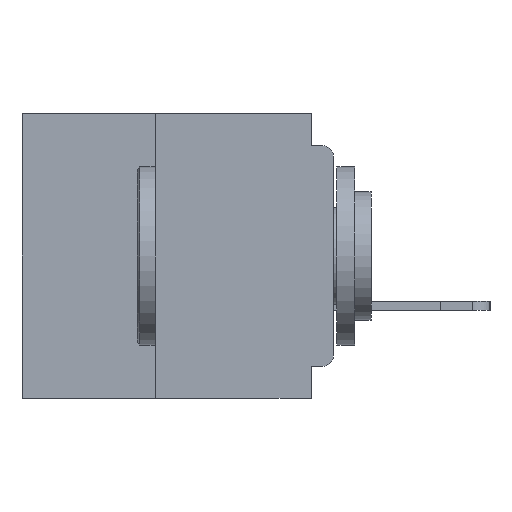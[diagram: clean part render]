
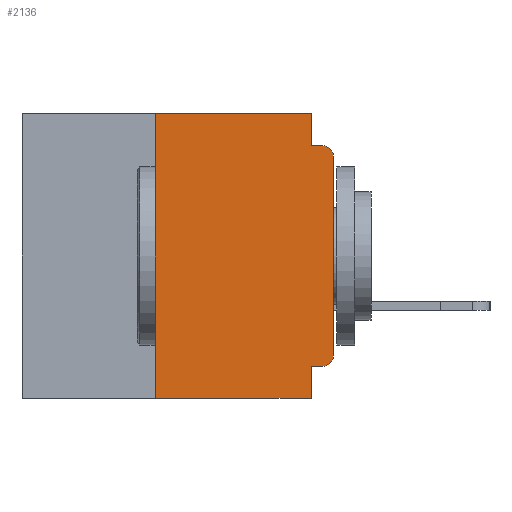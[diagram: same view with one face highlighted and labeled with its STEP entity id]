
A CAD part, left-side view. The second image highlights one B-rep face of the part: STEP entity #2136.
In plain terms, the highlighted planar face has unit normal (-1, 0, 0).
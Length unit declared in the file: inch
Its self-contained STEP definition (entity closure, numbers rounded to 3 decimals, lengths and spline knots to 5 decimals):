
#831 = LINE ( 'NONE', #15381, #50218 ) ;
#1664 = EDGE_CURVE ( 'NONE', #14596, #16155, #32058, .T. ) ;
#2136 = ADVANCED_FACE ( 'NONE', ( #37481 ), #32467, .F. ) ;
#2362 = VERTEX_POINT ( 'NONE', #25327 ) ;
#2366 = CARTESIAN_POINT ( 'NONE',  ( 0., 0.015, -0.355 ) ) ;
#2578 = EDGE_CURVE ( 'NONE', #16155, #28811, #19187, .T. ) ;
#3343 = AXIS2_PLACEMENT_3D ( 'NONE', #37265, #13981, #41214 ) ;
#3678 = ORIENTED_EDGE ( 'NONE', *, *, #29369, .F. ) ;
#4217 = VECTOR ( 'NONE', #15801, 39.37008 ) ;
#6455 = EDGE_CURVE ( 'NONE', #28859, #28811, #13585, .T. ) ;
#6988 = EDGE_CURVE ( 'NONE', #14596, #2362, #22668, .T. ) ;
#7192 = ORIENTED_EDGE ( 'NONE', *, *, #6988, .T. ) ;
#7932 = CARTESIAN_POINT ( 'NONE',  ( 0., 0., 0. ) ) ;
#10696 = CARTESIAN_POINT ( 'NONE',  ( 0., 0.25, 0. ) ) ;
#10801 = VERTEX_POINT ( 'NONE', #24145 ) ;
#12001 = CARTESIAN_POINT ( 'NONE',  ( 0., 0.031, -0.045 ) ) ;
#12273 = DIRECTION ( 'NONE',  ( 0., 0., 1. ) ) ;
#12374 = CARTESIAN_POINT ( 'NONE',  ( 0., 0.031, -0.355 ) ) ;
#12497 = VERTEX_POINT ( 'NONE', #31125 ) ;
#13357 = DIRECTION ( 'NONE',  ( 0., -1., 0. ) ) ;
#13410 = ORIENTED_EDGE ( 'NONE', *, *, #27637, .T. ) ;
#13585 = LINE ( 'NONE', #45611, #16021 ) ;
#13981 = DIRECTION ( 'NONE',  ( -1., 0., 0. ) ) ;
#13980 = VECTOR ( 'NONE', #22841, 39.37008 ) ;
#14596 = VERTEX_POINT ( 'NONE', #2366 ) ;
#14683 = LINE ( 'NONE', #7932, #4217 ) ;
#14730 = ORIENTED_EDGE ( 'NONE', *, *, #19282, .T. ) ;
#14836 = CARTESIAN_POINT ( 'NONE',  ( 0., 0.031, -0.4 ) ) ;
#15078 = ORIENTED_EDGE ( 'NONE', *, *, #1664, .F. ) ;
#15176 = CARTESIAN_POINT ( 'NONE',  ( 0., 0.25, -0.4 ) ) ;
#15381 = CARTESIAN_POINT ( 'NONE',  ( 0., 0., -0.045 ) ) ;
#15528 = EDGE_CURVE ( 'NONE', #28859, #43938, #20409, .T. ) ;
#15801 = DIRECTION ( 'NONE',  ( 0., 0., 1. ) ) ;
#16021 = VECTOR ( 'NONE', #26297, 39.37008 ) ;
#16155 = VERTEX_POINT ( 'NONE', #12374 ) ;
#19187 = LINE ( 'NONE', #20454, #20406 ) ;
#19282 = EDGE_CURVE ( 'NONE', #10801, #12497, #20714, .T. ) ;
#20397 = DIRECTION ( 'NONE',  ( 0., 0., -1. ) ) ;
#20406 = VECTOR ( 'NONE', #20397, 39.37008 ) ;
#20409 = LINE ( 'NONE', #35564, #50112 ) ;
#20454 = CARTESIAN_POINT ( 'NONE',  ( 0., 0.031, -0.4 ) ) ;
#20714 = CIRCLE ( 'NONE', #37743, 0.015 ) ;
#20836 = CARTESIAN_POINT ( 'NONE',  ( 0., 0.031, 0. ) ) ;
#21738 = VECTOR ( 'NONE', #45431, 39.37008 ) ;
#22668 = CIRCLE ( 'NONE', #3343, 0.015 ) ;
#22841 = DIRECTION ( 'NONE',  ( 0., 0., -1. ) ) ;
#23389 = DIRECTION ( 'NONE',  ( -1., 0., 0. ) ) ;
#24144 = VECTOR ( 'NONE', #13357, 39.37008 ) ;
#24145 = CARTESIAN_POINT ( 'NONE',  ( 0., 0., -0.06 ) ) ;
#25327 = CARTESIAN_POINT ( 'NONE',  ( 0., 0., -0.34 ) ) ;
#25545 = LINE ( 'NONE', #38298, #13980 ) ;
#26297 = DIRECTION ( 'NONE',  ( 0., -1., 0. ) ) ;
#27637 = EDGE_CURVE ( 'NONE', #2362, #10801, #14683, .T. ) ;
#28310 = VERTEX_POINT ( 'NONE', #12001 ) ;
#28811 = VERTEX_POINT ( 'NONE', #14836 ) ;
#28859 = VERTEX_POINT ( 'NONE', #15176 ) ;
#29369 = EDGE_CURVE ( 'NONE', #28310, #12497, #831, .T. ) ;
#30233 = ORIENTED_EDGE ( 'NONE', *, *, #6455, .T. ) ;
#30963 = ORIENTED_EDGE ( 'NONE', *, *, #15528, .F. ) ;
#31125 = CARTESIAN_POINT ( 'NONE',  ( 0., 0.015, -0.045 ) ) ;
#31317 = VERTEX_POINT ( 'NONE', #20836 ) ;
#32016 = DIRECTION ( 'NONE',  ( 0., 0., -1. ) ) ;
#32058 = LINE ( 'NONE', #45601, #21738 ) ;
#32074 = DIRECTION ( 'NONE',  ( 1., 0., 0. ) ) ;
#32134 = CARTESIAN_POINT ( 'NONE',  ( 0., 0.437, 0. ) ) ;
#32467 = PLANE ( 'NONE',  #42732 ) ;
#34395 = ORIENTED_EDGE ( 'NONE', *, *, #41054, .F. ) ;
#35564 = CARTESIAN_POINT ( 'NONE',  ( 0., 0.25, -0.4 ) ) ;
#36477 = CARTESIAN_POINT ( 'NONE',  ( 0., 0.437, 0. ) ) ;
#37265 = CARTESIAN_POINT ( 'NONE',  ( 0., 0.015, -0.34 ) ) ;
#37481 = FACE_OUTER_BOUND ( 'NONE', #44900, .T. ) ;
#37743 = AXIS2_PLACEMENT_3D ( 'NONE', #46630, #23389, #50496 ) ;
#38196 = ORIENTED_EDGE ( 'NONE', *, *, #2578, .F. ) ;
#38298 = CARTESIAN_POINT ( 'NONE',  ( 0., 0.031, 0. ) ) ;
#41054 = EDGE_CURVE ( 'NONE', #43938, #31317, #46011, .T. ) ;
#41214 = DIRECTION ( 'NONE',  ( 0., 0., -1. ) ) ;
#42732 = AXIS2_PLACEMENT_3D ( 'NONE', #32134, #32074, #32016 ) ;
#43938 = VERTEX_POINT ( 'NONE', #10696 ) ;
#44900 = EDGE_LOOP ( 'NONE', ( #13410, #14730, #3678, #47966, #34395, #30963, #30233, #38196, #15078, #7192 ) ) ;
#45079 = EDGE_CURVE ( 'NONE', #31317, #28310, #25545, .T. ) ;
#45431 = DIRECTION ( 'NONE',  ( 0., 1., 0. ) ) ;
#45601 = CARTESIAN_POINT ( 'NONE',  ( 0., 0., -0.355 ) ) ;
#45611 = CARTESIAN_POINT ( 'NONE',  ( 0., 0.437, -0.4 ) ) ;
#46011 = LINE ( 'NONE', #36477, #24144 ) ;
#46445 = DIRECTION ( 'NONE',  ( 0., -1., 0. ) ) ;
#46630 = CARTESIAN_POINT ( 'NONE',  ( 0., 0.015, -0.06 ) ) ;
#47966 = ORIENTED_EDGE ( 'NONE', *, *, #45079, .F. ) ;
#50112 = VECTOR ( 'NONE', #12273, 39.37008 ) ;
#50218 = VECTOR ( 'NONE', #46445, 39.37008 ) ;
#50496 = DIRECTION ( 'NONE',  ( 0., 0., -1. ) ) ;
